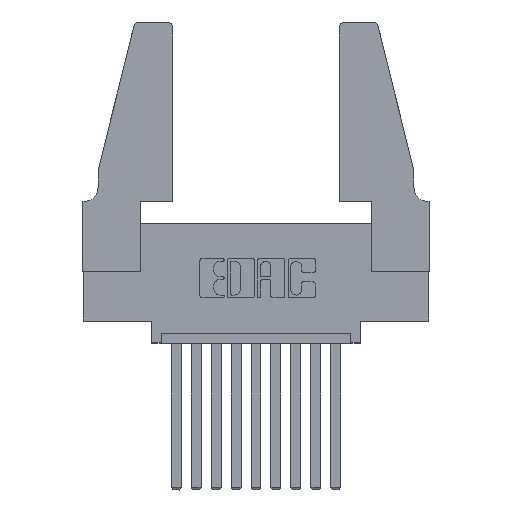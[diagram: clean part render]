
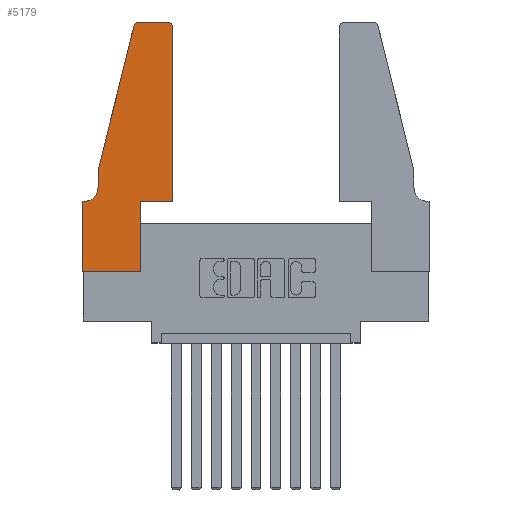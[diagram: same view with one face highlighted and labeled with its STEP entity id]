
A CAD part, top view. The second image highlights one B-rep face of the part: STEP entity #5179.
In plain terms, the highlighted planar face has unit normal (0, 0, 1).
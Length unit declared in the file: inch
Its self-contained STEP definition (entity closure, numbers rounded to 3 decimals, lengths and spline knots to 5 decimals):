
#320 = CARTESIAN_POINT ( 'NONE',  ( 0., 0.35, 0.37 ) ) ;
#406 = EDGE_CURVE ( 'NONE', #3067, #8941, #2942, .T. ) ;
#452 = VERTEX_POINT ( 'NONE', #1919 ) ;
#472 = VECTOR ( 'NONE', #4160, 39.37008 ) ;
#485 = EDGE_CURVE ( 'NONE', #12919, #13158, #3262, .T. ) ;
#875 = EDGE_CURVE ( 'NONE', #1547, #452, #10175, .T. ) ;
#1005 = VECTOR ( 'NONE', #10768, 39.37008 ) ;
#1146 = ORIENTED_EDGE ( 'NONE', *, *, #2850, .T. ) ;
#1175 = CARTESIAN_POINT ( 'NONE',  ( 0.4505, 0.35, 0.37 ) ) ;
#1210 = EDGE_CURVE ( 'NONE', #8941, #12054, #3083, .T. ) ;
#1223 = VECTOR ( 'NONE', #2509, 39.37008 ) ;
#1545 = DIRECTION ( 'NONE',  ( 1., 0., 0. ) ) ;
#1547 = VERTEX_POINT ( 'NONE', #8590 ) ;
#1599 = ORIENTED_EDGE ( 'NONE', *, *, #10087, .T. ) ;
#1919 = CARTESIAN_POINT ( 'NONE',  ( 0.4205, 1.25, 0.37 ) ) ;
#1974 = PLANE ( 'NONE',  #2243 ) ;
#2243 = AXIS2_PLACEMENT_3D ( 'NONE', #320, #7671, #1545 ) ;
#2246 = VERTEX_POINT ( 'NONE', #7164 ) ;
#2263 = LINE ( 'NONE', #2899, #472 ) ;
#2509 = DIRECTION ( 'NONE',  ( 1., 0., 0. ) ) ;
#2561 = FACE_OUTER_BOUND ( 'NONE', #12219, .T. ) ;
#2678 = VERTEX_POINT ( 'NONE', #5742 ) ;
#2850 = EDGE_CURVE ( 'NONE', #2678, #7354, #2953, .T. ) ;
#2883 = EDGE_CURVE ( 'NONE', #2246, #2678, #12882, .T. ) ;
#2899 = CARTESIAN_POINT ( 'NONE',  ( 0.2865, 0.35, 0.37 ) ) ;
#2942 = CIRCLE ( 'NONE', #8160, 0.03 ) ;
#2953 = LINE ( 'NONE', #4183, #5529 ) ;
#3067 = VERTEX_POINT ( 'NONE', #9745 ) ;
#3083 = LINE ( 'NONE', #7905, #5182 ) ;
#3194 = DIRECTION ( 'NONE',  ( 0., 1., 0. ) ) ;
#3219 = ORIENTED_EDGE ( 'NONE', *, *, #1210, .T. ) ;
#3262 = LINE ( 'NONE', #9548, #11938 ) ;
#3302 = LINE ( 'NONE', #5300, #7804 ) ;
#3389 = LINE ( 'NONE', #8376, #5490 ) ;
#3768 = DIRECTION ( 'NONE',  ( 0., 0., 1. ) ) ;
#3842 = EDGE_CURVE ( 'NONE', #13158, #1547, #3389, .T. ) ;
#4160 = DIRECTION ( 'NONE',  ( 0., 1., 0. ) ) ;
#4183 = CARTESIAN_POINT ( 'NONE',  ( 0.0755, 0.35, 0.37 ) ) ;
#4189 = AXIS2_PLACEMENT_3D ( 'NONE', #5287, #7423, #12457 ) ;
#4236 = CARTESIAN_POINT ( 'NONE',  ( 0., 0.35, 0.37 ) ) ;
#5179 = ADVANCED_FACE ( 'NONE', ( #2561 ), #1974, .T. ) ;
#5182 = VECTOR ( 'NONE', #13035, 39.37008 ) ;
#5287 = CARTESIAN_POINT ( 'NONE',  ( 0.4205, 1.22, 0.37 ) ) ;
#5300 = CARTESIAN_POINT ( 'NONE',  ( 0.2605, 1.25, 0.37 ) ) ;
#5490 = VECTOR ( 'NONE', #3194, 39.37008 ) ;
#5529 = VECTOR ( 'NONE', #11365, 39.37008 ) ;
#5599 = ORIENTED_EDGE ( 'NONE', *, *, #406, .T. ) ;
#5742 = CARTESIAN_POINT ( 'NONE',  ( 0.0055, 0.35, 0.37 ) ) ;
#5760 = LINE ( 'NONE', #7685, #1223 ) ;
#5813 = CARTESIAN_POINT ( 'NONE',  ( 0.0755, 0.5, 0.37 ) ) ;
#5853 = AXIS2_PLACEMENT_3D ( 'NONE', #11675, #8619, #7552 ) ;
#5932 = DIRECTION ( 'NONE',  ( 1., 0., 0. ) ) ;
#6157 = EDGE_CURVE ( 'NONE', #7314, #12843, #5760, .T. ) ;
#6206 = VECTOR ( 'NONE', #12043, 39.37008 ) ;
#6491 = LINE ( 'NONE', #9602, #1005 ) ;
#6671 = LINE ( 'NONE', #8111, #6206 ) ;
#7164 = CARTESIAN_POINT ( 'NONE',  ( 0.0755, 0.42, 0.37 ) ) ;
#7252 = CARTESIAN_POINT ( 'NONE',  ( 0.2865, 0.35, 0.37 ) ) ;
#7314 = VERTEX_POINT ( 'NONE', #10525 ) ;
#7354 = VERTEX_POINT ( 'NONE', #4236 ) ;
#7423 = DIRECTION ( 'NONE',  ( 0., 0., 1. ) ) ;
#7508 = ORIENTED_EDGE ( 'NONE', *, *, #485, .T. ) ;
#7552 = DIRECTION ( 'NONE',  ( -1., 0., 0. ) ) ;
#7671 = DIRECTION ( 'NONE',  ( 0., 0., 1. ) ) ;
#7685 = CARTESIAN_POINT ( 'NONE',  ( 0., 0., 0.37 ) ) ;
#7713 = EDGE_CURVE ( 'NONE', #7354, #7314, #6671, .T. ) ;
#7804 = VECTOR ( 'NONE', #12513, 39.37008 ) ;
#7905 = CARTESIAN_POINT ( 'NONE',  ( 0.0755, 0.5, 0.37 ) ) ;
#8111 = CARTESIAN_POINT ( 'NONE',  ( 0., 0., 0.37 ) ) ;
#8160 = AXIS2_PLACEMENT_3D ( 'NONE', #12070, #3768, #5932 ) ;
#8274 = ORIENTED_EDGE ( 'NONE', *, *, #3842, .T. ) ;
#8376 = CARTESIAN_POINT ( 'NONE',  ( 0.4505, 0.35, 0.37 ) ) ;
#8434 = ORIENTED_EDGE ( 'NONE', *, *, #8994, .T. ) ;
#8529 = CARTESIAN_POINT ( 'NONE',  ( 0.25487, 1.22718, 0.37 ) ) ;
#8590 = CARTESIAN_POINT ( 'NONE',  ( 0.4505, 1.22, 0.37 ) ) ;
#8619 = DIRECTION ( 'NONE',  ( 0., 0., -1. ) ) ;
#8941 = VERTEX_POINT ( 'NONE', #8529 ) ;
#8994 = EDGE_CURVE ( 'NONE', #452, #3067, #3302, .T. ) ;
#9179 = ORIENTED_EDGE ( 'NONE', *, *, #11763, .T. ) ;
#9548 = CARTESIAN_POINT ( 'NONE',  ( 0.4505, 0.35, 0.37 ) ) ;
#9602 = CARTESIAN_POINT ( 'NONE',  ( 0.0755, 0.5, 0.37 ) ) ;
#9638 = ORIENTED_EDGE ( 'NONE', *, *, #875, .T. ) ;
#9745 = CARTESIAN_POINT ( 'NONE',  ( 0.284, 1.25, 0.37 ) ) ;
#10087 = EDGE_CURVE ( 'NONE', #12054, #2246, #6491, .T. ) ;
#10175 = CIRCLE ( 'NONE', #4189, 0.03 ) ;
#10525 = CARTESIAN_POINT ( 'NONE',  ( 0., 0., 0.37 ) ) ;
#10768 = DIRECTION ( 'NONE',  ( 0., -1., 0. ) ) ;
#10997 = ORIENTED_EDGE ( 'NONE', *, *, #7713, .T. ) ;
#11365 = DIRECTION ( 'NONE',  ( -1., 0., 0. ) ) ;
#11413 = ORIENTED_EDGE ( 'NONE', *, *, #6157, .T. ) ;
#11607 = DIRECTION ( 'NONE',  ( 1., 0., 0. ) ) ;
#11675 = CARTESIAN_POINT ( 'NONE',  ( 0.0055, 0.42, 0.37 ) ) ;
#11691 = ORIENTED_EDGE ( 'NONE', *, *, #2883, .T. ) ;
#11763 = EDGE_CURVE ( 'NONE', #12843, #12919, #2263, .T. ) ;
#11938 = VECTOR ( 'NONE', #11607, 39.37008 ) ;
#12043 = DIRECTION ( 'NONE',  ( 0., -1., 0. ) ) ;
#12054 = VERTEX_POINT ( 'NONE', #5813 ) ;
#12070 = CARTESIAN_POINT ( 'NONE',  ( 0.284, 1.22, 0.37 ) ) ;
#12073 = CARTESIAN_POINT ( 'NONE',  ( 0.2865, 0., 0.37 ) ) ;
#12219 = EDGE_LOOP ( 'NONE', ( #8434, #5599, #3219, #1599, #11691, #1146, #10997, #11413, #9179, #7508, #8274, #9638 ) ) ;
#12457 = DIRECTION ( 'NONE',  ( 1., 0., 0. ) ) ;
#12513 = DIRECTION ( 'NONE',  ( -1., 0., 0. ) ) ;
#12843 = VERTEX_POINT ( 'NONE', #12073 ) ;
#12882 = CIRCLE ( 'NONE', #5853, 0.07 ) ;
#12919 = VERTEX_POINT ( 'NONE', #7252 ) ;
#13035 = DIRECTION ( 'NONE',  ( -0.239, -0.971, 0. ) ) ;
#13158 = VERTEX_POINT ( 'NONE', #1175 ) ;
